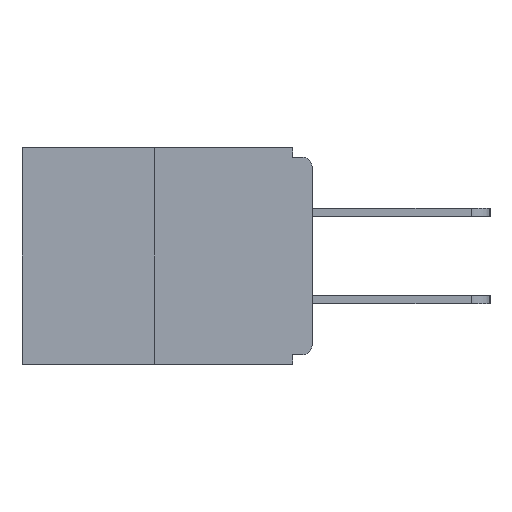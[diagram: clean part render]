
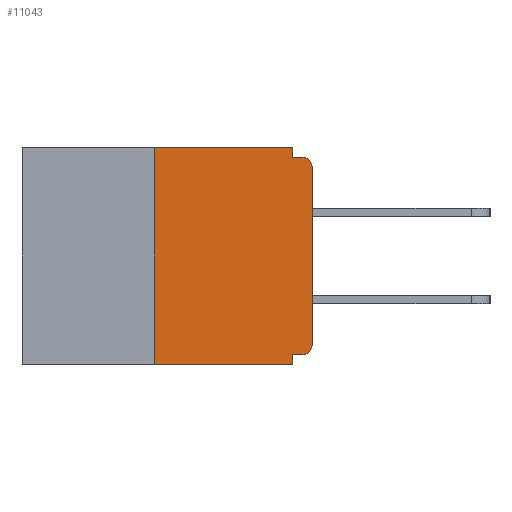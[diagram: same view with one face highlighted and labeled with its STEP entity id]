
A CAD part, left-side view. The second image highlights one B-rep face of the part: STEP entity #11043.
In plain terms, the highlighted planar face has unit normal (-1, 0, 0).
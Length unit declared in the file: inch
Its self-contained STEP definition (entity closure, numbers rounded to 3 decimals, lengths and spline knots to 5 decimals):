
#352 = CARTESIAN_POINT ( 'NONE',  ( 0., 0.25, 0. ) ) ;
#494 = LINE ( 'NONE', #16519, #3366 ) ;
#510 = DIRECTION ( 'NONE',  ( 0., 0., 1. ) ) ;
#1216 = ORIENTED_EDGE ( 'NONE', *, *, #20296, .F. ) ;
#1432 = DIRECTION ( 'NONE',  ( 0., 0., 1. ) ) ;
#1456 = AXIS2_PLACEMENT_3D ( 'NONE', #5915, #17146, #28502 ) ;
#1562 = VERTEX_POINT ( 'NONE', #12983 ) ;
#1651 = ORIENTED_EDGE ( 'NONE', *, *, #27732, .T. ) ;
#1663 = CARTESIAN_POINT ( 'NONE',  ( 0., 0.46, -0.343 ) ) ;
#2506 = CARTESIAN_POINT ( 'NONE',  ( 0., 0.031, -0.343 ) ) ;
#2638 = CARTESIAN_POINT ( 'NONE',  ( 0., 0., -0.328 ) ) ;
#3207 = CARTESIAN_POINT ( 'NONE',  ( 0., 0.031, -0.343 ) ) ;
#3366 = VECTOR ( 'NONE', #9631, 39.37008 ) ;
#4785 = EDGE_CURVE ( 'NONE', #11681, #1562, #494, .T. ) ;
#5313 = LINE ( 'NONE', #2638, #18152 ) ;
#5598 = DIRECTION ( 'NONE',  ( 0., 0., -1. ) ) ;
#5915 = CARTESIAN_POINT ( 'NONE',  ( 0., 0.015, -0.313 ) ) ;
#6405 = VERTEX_POINT ( 'NONE', #26920 ) ;
#6469 = DIRECTION ( 'NONE',  ( 0., 0., -1. ) ) ;
#6657 = CARTESIAN_POINT ( 'NONE',  ( 0., 0.015, -0.328 ) ) ;
#6708 = ORIENTED_EDGE ( 'NONE', *, *, #23583, .F. ) ;
#6893 = VERTEX_POINT ( 'NONE', #19039 ) ;
#6970 = DIRECTION ( 'NONE',  ( 0., 1., 0. ) ) ;
#7464 = VECTOR ( 'NONE', #510, 39.37008 ) ;
#7948 = ORIENTED_EDGE ( 'NONE', *, *, #16463, .T. ) ;
#8088 = VECTOR ( 'NONE', #5598, 39.37008 ) ;
#8951 = ORIENTED_EDGE ( 'NONE', *, *, #23209, .F. ) ;
#9144 = DIRECTION ( 'NONE',  ( 0., -1., 0. ) ) ;
#9396 = VECTOR ( 'NONE', #1432, 39.37008 ) ;
#9631 = DIRECTION ( 'NONE',  ( 0., -1., 0. ) ) ;
#9781 = EDGE_CURVE ( 'NONE', #6405, #10084, #27015, .T. ) ;
#9798 = LINE ( 'NONE', #19096, #18945 ) ;
#10084 = VERTEX_POINT ( 'NONE', #28346 ) ;
#11043 = ADVANCED_FACE ( 'NONE', ( #13889 ), #16560, .F. ) ;
#11109 = VERTEX_POINT ( 'NONE', #2506 ) ;
#11681 = VERTEX_POINT ( 'NONE', #26681 ) ;
#12467 = ORIENTED_EDGE ( 'NONE', *, *, #28238, .F. ) ;
#12983 = CARTESIAN_POINT ( 'NONE',  ( 0., 0.015, -0.015 ) ) ;
#13254 = CARTESIAN_POINT ( 'NONE',  ( 0., 0., 0. ) ) ;
#13530 = CARTESIAN_POINT ( 'NONE',  ( 0., 0.015, -0.03 ) ) ;
#13603 = ORIENTED_EDGE ( 'NONE', *, *, #4785, .F. ) ;
#13669 = DIRECTION ( 'NONE',  ( -1., 0., 0. ) ) ;
#13776 = DIRECTION ( 'NONE',  ( 0., -1., 0. ) ) ;
#13889 = FACE_OUTER_BOUND ( 'NONE', #15144, .T. ) ;
#14017 = LINE ( 'NONE', #352, #7464 ) ;
#14317 = DIRECTION ( 'NONE',  ( 0., 0., -1. ) ) ;
#14378 = CIRCLE ( 'NONE', #25337, 0.015 ) ;
#14398 = VERTEX_POINT ( 'NONE', #17190 ) ;
#14940 = EDGE_CURVE ( 'NONE', #10084, #1562, #14378, .T. ) ;
#15144 = EDGE_LOOP ( 'NONE', ( #8951, #6708, #7948, #1216, #28468, #1651, #25286, #19314, #13603, #12467 ) ) ;
#16463 = EDGE_CURVE ( 'NONE', #14398, #11109, #29050, .T. ) ;
#16519 = CARTESIAN_POINT ( 'NONE',  ( 0., 0., -0.015 ) ) ;
#16560 = PLANE ( 'NONE',  #18538 ) ;
#17146 = DIRECTION ( 'NONE',  ( -1., 0., 0. ) ) ;
#17190 = CARTESIAN_POINT ( 'NONE',  ( 0., 0.25, -0.343 ) ) ;
#18152 = VECTOR ( 'NONE', #6970, 39.37008 ) ;
#18237 = DIRECTION ( 'NONE',  ( 1., 0., 0. ) ) ;
#18538 = AXIS2_PLACEMENT_3D ( 'NONE', #27922, #18237, #14317 ) ;
#18945 = VECTOR ( 'NONE', #13776, 39.37008 ) ;
#19039 = CARTESIAN_POINT ( 'NONE',  ( 0., 0.031, -0.328 ) ) ;
#19096 = CARTESIAN_POINT ( 'NONE',  ( 0., 0.46, 0. ) ) ;
#19152 = CIRCLE ( 'NONE', #1456, 0.015 ) ;
#19225 = VERTEX_POINT ( 'NONE', #21376 ) ;
#19314 = ORIENTED_EDGE ( 'NONE', *, *, #14940, .T. ) ;
#20135 = EDGE_CURVE ( 'NONE', #20424, #6893, #5313, .T. ) ;
#20250 = DIRECTION ( 'NONE',  ( 0., 0., -1. ) ) ;
#20296 = EDGE_CURVE ( 'NONE', #6893, #11109, #25965, .T. ) ;
#20424 = VERTEX_POINT ( 'NONE', #6657 ) ;
#21019 = VECTOR ( 'NONE', #6469, 39.37008 ) ;
#21376 = CARTESIAN_POINT ( 'NONE',  ( 0., 0.031, 0. ) ) ;
#22913 = CARTESIAN_POINT ( 'NONE',  ( 0., 0.031, 0. ) ) ;
#23209 = EDGE_CURVE ( 'NONE', #25399, #19225, #9798, .T. ) ;
#23583 = EDGE_CURVE ( 'NONE', #14398, #25399, #14017, .T. ) ;
#24421 = CARTESIAN_POINT ( 'NONE',  ( 0., 0.25, 0. ) ) ;
#24713 = LINE ( 'NONE', #22913, #21019 ) ;
#25286 = ORIENTED_EDGE ( 'NONE', *, *, #9781, .T. ) ;
#25337 = AXIS2_PLACEMENT_3D ( 'NONE', #13530, #13669, #20250 ) ;
#25399 = VERTEX_POINT ( 'NONE', #24421 ) ;
#25965 = LINE ( 'NONE', #3207, #8088 ) ;
#26681 = CARTESIAN_POINT ( 'NONE',  ( 0., 0.031, -0.015 ) ) ;
#26920 = CARTESIAN_POINT ( 'NONE',  ( 0., 0., -0.313 ) ) ;
#27015 = LINE ( 'NONE', #13254, #9396 ) ;
#27732 = EDGE_CURVE ( 'NONE', #20424, #6405, #19152, .T. ) ;
#27922 = CARTESIAN_POINT ( 'NONE',  ( 0., 0.46, 0. ) ) ;
#28055 = VECTOR ( 'NONE', #9144, 39.37008 ) ;
#28238 = EDGE_CURVE ( 'NONE', #19225, #11681, #24713, .T. ) ;
#28346 = CARTESIAN_POINT ( 'NONE',  ( 0., 0., -0.03 ) ) ;
#28468 = ORIENTED_EDGE ( 'NONE', *, *, #20135, .F. ) ;
#28502 = DIRECTION ( 'NONE',  ( 0., 0., -1. ) ) ;
#29050 = LINE ( 'NONE', #1663, #28055 ) ;
